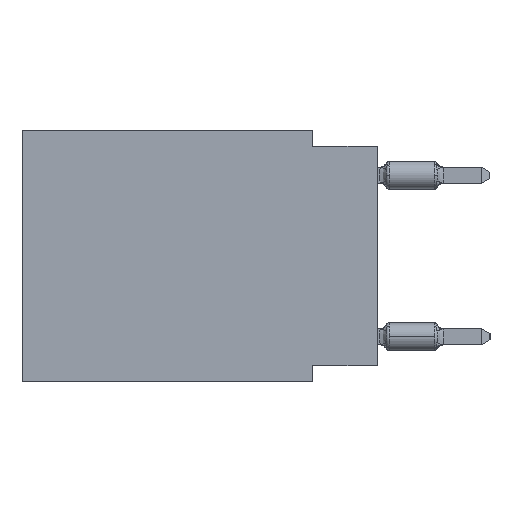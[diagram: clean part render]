
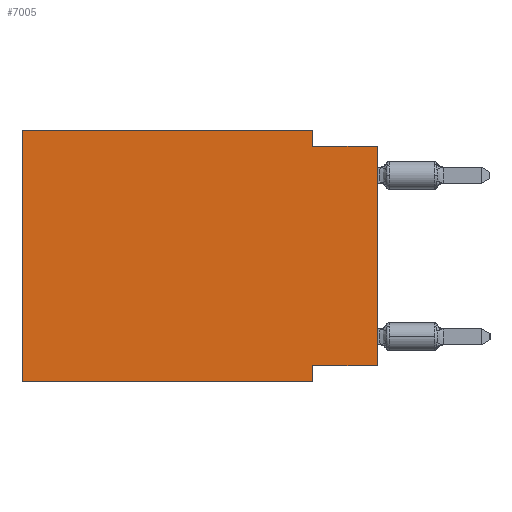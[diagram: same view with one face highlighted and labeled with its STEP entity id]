
A CAD part, left-side view. The second image highlights one B-rep face of the part: STEP entity #7005.
In plain terms, the highlighted planar face has unit normal (-1, 0, 0).
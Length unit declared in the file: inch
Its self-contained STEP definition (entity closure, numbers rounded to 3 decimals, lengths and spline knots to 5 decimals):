
#1918 = LINE ( 'NONE', #36908, #33824 ) ;
#2197 = ORIENTED_EDGE ( 'NONE', *, *, #48629, .F. ) ;
#2434 = CARTESIAN_POINT ( 'NONE',  ( 0., 0.55, 0. ) ) ;
#3291 = ORIENTED_EDGE ( 'NONE', *, *, #5542, .F. ) ;
#3967 = VECTOR ( 'NONE', #36605, 39.37008 ) ;
#4302 = VERTEX_POINT ( 'NONE', #16574 ) ;
#5011 = FACE_OUTER_BOUND ( 'NONE', #48239, .T. ) ;
#5542 = EDGE_CURVE ( 'NONE', #28039, #31164, #50559, .T. ) ;
#6036 = DIRECTION ( 'NONE',  ( 0., 0., 1. ) ) ;
#6404 = CARTESIAN_POINT ( 'NONE',  ( 0., 0.55, 0. ) ) ;
#7005 = ADVANCED_FACE ( 'NONE', ( #5011 ), #44591, .F. ) ;
#8654 = DIRECTION ( 'NONE',  ( 0., -1., 0. ) ) ;
#9603 = DIRECTION ( 'NONE',  ( 0., 1., 0. ) ) ;
#9886 = CARTESIAN_POINT ( 'NONE',  ( 0., 0.55, 0. ) ) ;
#10019 = EDGE_CURVE ( 'NONE', #11200, #17454, #1918, .T. ) ;
#10580 = VERTEX_POINT ( 'NONE', #30254 ) ;
#11200 = VERTEX_POINT ( 'NONE', #47113 ) ;
#11291 = ORIENTED_EDGE ( 'NONE', *, *, #40595, .F. ) ;
#13028 = CARTESIAN_POINT ( 'NONE',  ( 0., 0., -0.025 ) ) ;
#13485 = CARTESIAN_POINT ( 'NONE',  ( 0., 0.55, 0. ) ) ;
#15673 = VECTOR ( 'NONE', #22067, 39.37008 ) ;
#16050 = LINE ( 'NONE', #23984, #3967 ) ;
#16574 = CARTESIAN_POINT ( 'NONE',  ( 0., 0.1, -0.025 ) ) ;
#17454 = VERTEX_POINT ( 'NONE', #31793 ) ;
#19924 = DIRECTION ( 'NONE',  ( 0., 0., -1. ) ) ;
#22067 = DIRECTION ( 'NONE',  ( 0., -1., 0. ) ) ;
#22258 = ORIENTED_EDGE ( 'NONE', *, *, #10019, .T. ) ;
#23269 = CARTESIAN_POINT ( 'NONE',  ( 0., 0.1, 0. ) ) ;
#23984 = CARTESIAN_POINT ( 'NONE',  ( 0., 0.1, -0.39 ) ) ;
#24180 = CARTESIAN_POINT ( 'NONE',  ( 0., 0., -0.025 ) ) ;
#25465 = CARTESIAN_POINT ( 'NONE',  ( 0., 0.1, 0. ) ) ;
#25769 = CARTESIAN_POINT ( 'NONE',  ( 0., 0., -0.365 ) ) ;
#26100 = VERTEX_POINT ( 'NONE', #46479 ) ;
#26688 = ORIENTED_EDGE ( 'NONE', *, *, #50777, .F. ) ;
#26842 = DIRECTION ( 'NONE',  ( 0., 0., 1. ) ) ;
#27856 = EDGE_CURVE ( 'NONE', #31164, #4302, #39462, .T. ) ;
#28039 = VERTEX_POINT ( 'NONE', #9886 ) ;
#29212 = EDGE_CURVE ( 'NONE', #10580, #39587, #37151, .T. ) ;
#30254 = CARTESIAN_POINT ( 'NONE',  ( 0., 0., -0.365 ) ) ;
#31164 = VERTEX_POINT ( 'NONE', #25465 ) ;
#31793 = CARTESIAN_POINT ( 'NONE',  ( 0., 0.1, -0.39 ) ) ;
#32047 = VECTOR ( 'NONE', #6036, 39.37008 ) ;
#32527 = DIRECTION ( 'NONE',  ( 1., 0., 0. ) ) ;
#32553 = AXIS2_PLACEMENT_3D ( 'NONE', #13485, #32527, #44849 ) ;
#33820 = DIRECTION ( 'NONE',  ( 0., -1., 0. ) ) ;
#33824 = VECTOR ( 'NONE', #33820, 39.37008 ) ;
#34000 = VECTOR ( 'NONE', #26842, 39.37008 ) ;
#34834 = LINE ( 'NONE', #2434, #34000 ) ;
#36605 = DIRECTION ( 'NONE',  ( 0., 0., -1. ) ) ;
#36908 = CARTESIAN_POINT ( 'NONE',  ( 0., 0.55, -0.39 ) ) ;
#36933 = VECTOR ( 'NONE', #9603, 39.37008 ) ;
#37151 = LINE ( 'NONE', #45106, #32047 ) ;
#37324 = ORIENTED_EDGE ( 'NONE', *, *, #27856, .F. ) ;
#39462 = LINE ( 'NONE', #23269, #45986 ) ;
#39587 = VERTEX_POINT ( 'NONE', #24180 ) ;
#40595 = EDGE_CURVE ( 'NONE', #4302, #39587, #48978, .T. ) ;
#41985 = ORIENTED_EDGE ( 'NONE', *, *, #47288, .F. ) ;
#44591 = PLANE ( 'NONE',  #32553 ) ;
#44849 = DIRECTION ( 'NONE',  ( 0., 0., -1. ) ) ;
#45106 = CARTESIAN_POINT ( 'NONE',  ( 0., 0., 0. ) ) ;
#45308 = LINE ( 'NONE', #25769, #36933 ) ;
#45986 = VECTOR ( 'NONE', #19924, 39.37008 ) ;
#46479 = CARTESIAN_POINT ( 'NONE',  ( 0., 0.1, -0.365 ) ) ;
#46717 = ORIENTED_EDGE ( 'NONE', *, *, #29212, .T. ) ;
#47113 = CARTESIAN_POINT ( 'NONE',  ( 0., 0.55, -0.39 ) ) ;
#47288 = EDGE_CURVE ( 'NONE', #26100, #17454, #16050, .T. ) ;
#47962 = VECTOR ( 'NONE', #8654, 39.37008 ) ;
#48239 = EDGE_LOOP ( 'NONE', ( #46717, #11291, #37324, #3291, #26688, #22258, #41985, #2197 ) ) ;
#48629 = EDGE_CURVE ( 'NONE', #10580, #26100, #45308, .T. ) ;
#48978 = LINE ( 'NONE', #13028, #47962 ) ;
#50559 = LINE ( 'NONE', #6404, #15673 ) ;
#50777 = EDGE_CURVE ( 'NONE', #11200, #28039, #34834, .T. ) ;
